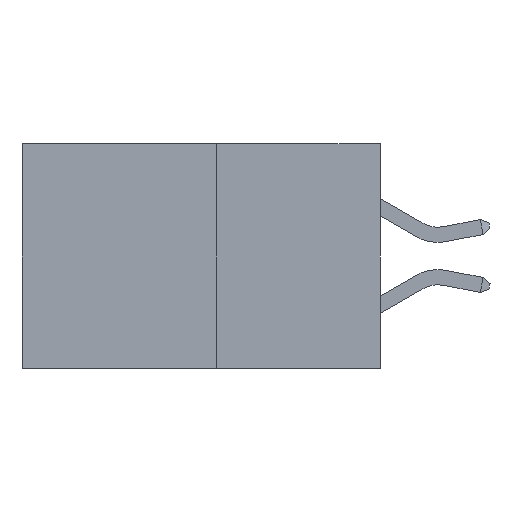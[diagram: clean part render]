
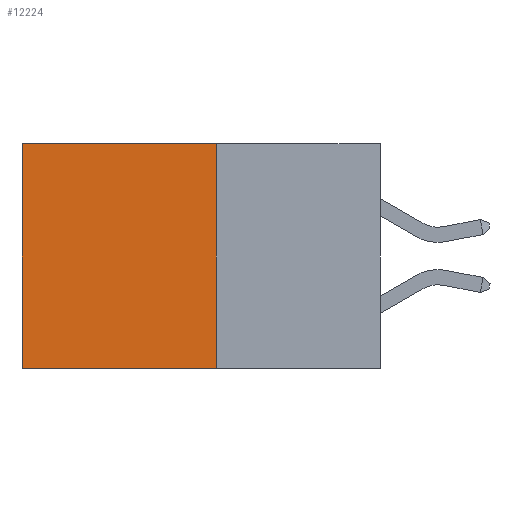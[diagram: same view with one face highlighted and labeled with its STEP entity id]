
A CAD part, left-side view. The second image highlights one B-rep face of the part: STEP entity #12224.
In plain terms, the highlighted planar face has unit normal (-1, 0, 0).
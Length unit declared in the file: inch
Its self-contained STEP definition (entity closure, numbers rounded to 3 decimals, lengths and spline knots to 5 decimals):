
#26 = AXIS2_PLACEMENT_3D ( 'NONE', #3770, #21647, #6340 ) ;
#2514 = EDGE_CURVE ( 'NONE', #10621, #23338, #32800, .T. ) ;
#2582 = VECTOR ( 'NONE', #8241, 39.37008 ) ;
#3770 = CARTESIAN_POINT ( 'NONE',  ( 0.277, 0.27, -0.37 ) ) ;
#4231 = EDGE_LOOP ( 'NONE', ( #11401, #16221, #15050, #8400 ) ) ;
#5694 = CARTESIAN_POINT ( 'NONE',  ( 0.277, 0.59, -0.37 ) ) ;
#6340 = DIRECTION ( 'NONE',  ( 0., 0., -1. ) ) ;
#6622 = EDGE_CURVE ( 'NONE', #24802, #23338, #24466, .T. ) ;
#8241 = DIRECTION ( 'NONE',  ( 0., 1., 0. ) ) ;
#8400 = ORIENTED_EDGE ( 'NONE', *, *, #10671, .T. ) ;
#9388 = LINE ( 'NONE', #31012, #2582 ) ;
#9986 = VECTOR ( 'NONE', #18792, 39.37008 ) ;
#10621 = VERTEX_POINT ( 'NONE', #30904 ) ;
#10671 = EDGE_CURVE ( 'NONE', #24956, #10621, #9388, .T. ) ;
#11401 = ORIENTED_EDGE ( 'NONE', *, *, #2514, .T. ) ;
#12224 = ADVANCED_FACE ( 'NONE', ( #18863 ), #19084, .F. ) ;
#13430 = EDGE_CURVE ( 'NONE', #24956, #24802, #16778, .T. ) ;
#13670 = CARTESIAN_POINT ( 'NONE',  ( 0.277, 0.27, -0.37 ) ) ;
#15050 = ORIENTED_EDGE ( 'NONE', *, *, #13430, .F. ) ;
#16221 = ORIENTED_EDGE ( 'NONE', *, *, #6622, .F. ) ;
#16379 = DIRECTION ( 'NONE',  ( 0., 0., -1. ) ) ;
#16778 = LINE ( 'NONE', #13670, #9986 ) ;
#18481 = VECTOR ( 'NONE', #23470, 39.37008 ) ;
#18792 = DIRECTION ( 'NONE',  ( 0., 0., -1. ) ) ;
#18863 = FACE_OUTER_BOUND ( 'NONE', #4231, .T. ) ;
#19084 = PLANE ( 'NONE',  #26 ) ;
#19142 = CARTESIAN_POINT ( 'NONE',  ( 0.277, 0.59, -0.37 ) ) ;
#19404 = VECTOR ( 'NONE', #16379, 39.37008 ) ;
#21647 = DIRECTION ( 'NONE',  ( 1., 0., 0. ) ) ;
#21841 = CARTESIAN_POINT ( 'NONE',  ( 0.277, 0.27, -0.37 ) ) ;
#22395 = CARTESIAN_POINT ( 'NONE',  ( 0.277, 0.27, 0. ) ) ;
#23338 = VERTEX_POINT ( 'NONE', #5694 ) ;
#23470 = DIRECTION ( 'NONE',  ( 0., 1., 0. ) ) ;
#23572 = CARTESIAN_POINT ( 'NONE',  ( 0.277, 0.27, -0.37 ) ) ;
#24466 = LINE ( 'NONE', #23572, #18481 ) ;
#24802 = VERTEX_POINT ( 'NONE', #21841 ) ;
#24956 = VERTEX_POINT ( 'NONE', #22395 ) ;
#30904 = CARTESIAN_POINT ( 'NONE',  ( 0.277, 0.59, 0. ) ) ;
#31012 = CARTESIAN_POINT ( 'NONE',  ( 0.277, 0.27, 0. ) ) ;
#32800 = LINE ( 'NONE', #19142, #19404 ) ;
